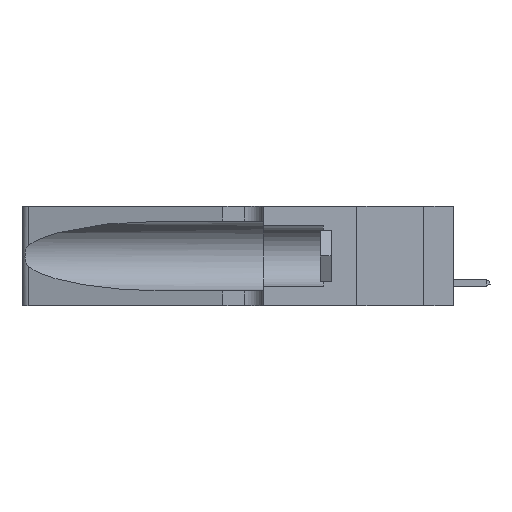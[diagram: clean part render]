
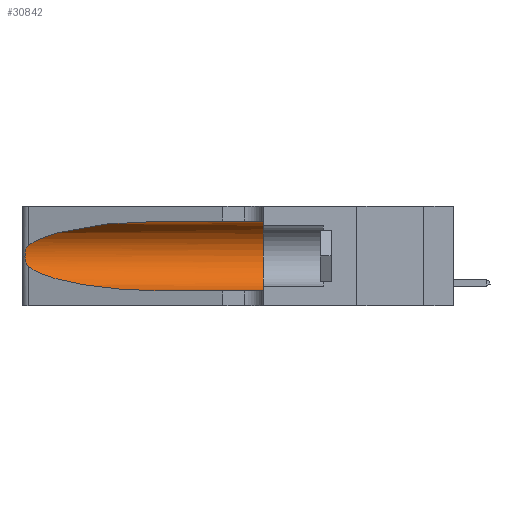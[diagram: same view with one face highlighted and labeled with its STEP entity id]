
A CAD part, left-side view. The second image highlights one B-rep face of the part: STEP entity #30842.
In plain terms, the highlighted cylindrical face has radius 3.308 mm (diameter 6.617 mm), a partial arc.
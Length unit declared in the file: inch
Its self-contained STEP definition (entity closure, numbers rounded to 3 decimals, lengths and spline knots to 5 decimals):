
#188 =( BOUNDED_CURVE ( )  B_SPLINE_CURVE ( 3, ( #22121, #29114, #4600, #29251 ),
 .UNSPECIFIED., .F., .F. ) 
 B_SPLINE_CURVE_WITH_KNOTS ( ( 4, 4 ),
 ( 3.44316, 4.71239 ),
 .UNSPECIFIED. ) 
 CURVE ( )  GEOMETRIC_REPRESENTATION_ITEM ( )  RATIONAL_B_SPLINE_CURVE ( ( 1., 0.87, 0.87, 1. ) ) 
 REPRESENTATION_ITEM ( '' )  );
#1077 = CARTESIAN_POINT ( 'NONE',  ( 0.25487, 1.22718, 0.22369 ) ) ;
#1195 = CYLINDRICAL_SURFACE ( 'NONE', #4130, 0.13025 ) ;
#1850 = CARTESIAN_POINT ( 'NONE',  ( 0.1305, 0.35, 0.31525 ) ) ;
#2791 = ORIENTED_EDGE ( 'NONE', *, *, #32027, .T. ) ;
#3034 = CARTESIAN_POINT ( 'NONE',  ( 0.25487, 1.22718, 0.14631 ) ) ;
#3228 = B_SPLINE_CURVE_WITH_KNOTS ( 'NONE', 3,
 ( #8041, #13827, #14368, #7908, #35420, #29452, #14245, #26494, #29583, #11113, #35843, #17309, #5080, #26637 ),
 .UNSPECIFIED., .F., .F.,
 ( 4, 2, 2, 2, 2, 2, 4 ),
 ( 0., 0.00027, 0.00053, 0.00107, 0.0016, 0.00187, 0.00214 ),
 .UNSPECIFIED. ) ;
#3767 = VERTEX_POINT ( 'NONE', #1850 ) ;
#4130 = AXIS2_PLACEMENT_3D ( 'NONE', #20902, #27401, #15110 ) ;
#4600 = CARTESIAN_POINT ( 'NONE',  ( 0.18966, 0.96281, 0.05475 ) ) ;
#5080 = CARTESIAN_POINT ( 'NONE',  ( 0.25555, 1.22993, 0.14849 ) ) ;
#5114 = EDGE_CURVE ( 'NONE', #3767, #33739, #23675, .T. ) ;
#5164 = CARTESIAN_POINT ( 'NONE',  ( 0.1305, 0.72297, 0.31525 ) ) ;
#5183 = CARTESIAN_POINT ( 'NONE',  ( 0.1305, 1.61858, 0.31525 ) ) ;
#5314 = DIRECTION ( 'NONE',  ( 0., -1., 0. ) ) ;
#5830 = AXIS2_PLACEMENT_3D ( 'NONE', #5868, #37039, #36783 ) ;
#5868 = CARTESIAN_POINT ( 'NONE',  ( 0.1305, 0.35, 0.185 ) ) ;
#7737 = ORIENTED_EDGE ( 'NONE', *, *, #20285, .F. ) ;
#7805 = EDGE_LOOP ( 'NONE', ( #2791, #36984, #19029, #29726, #11696, #7737 ) ) ;
#7908 = CARTESIAN_POINT ( 'NONE',  ( 0.25787, 1.23484, 0.2124 ) ) ;
#8041 = CARTESIAN_POINT ( 'NONE',  ( 0.25487, 1.22718, 0.22369 ) ) ;
#11113 = CARTESIAN_POINT ( 'NONE',  ( 0.25856, 1.23593, 0.16098 ) ) ;
#11696 = ORIENTED_EDGE ( 'NONE', *, *, #5114, .F. ) ;
#13827 = CARTESIAN_POINT ( 'NONE',  ( 0.25555, 1.22994, 0.2215 ) ) ;
#14245 = CARTESIAN_POINT ( 'NONE',  ( 0.26075, 1.23896, 0.19203 ) ) ;
#14368 = CARTESIAN_POINT ( 'NONE',  ( 0.25639, 1.23184, 0.21858 ) ) ;
#14747 = VECTOR ( 'NONE', #22527, 39.37008 ) ;
#14968 = CARTESIAN_POINT ( 'NONE',  ( 0.18966, 0.96281, 0.31525 ) ) ;
#15110 = DIRECTION ( 'NONE',  ( 0., 0., -1. ) ) ;
#15194 = LINE ( 'NONE', #20760, #14747 ) ;
#15802 = VECTOR ( 'NONE', #5314, 39.37008 ) ;
#17309 = CARTESIAN_POINT ( 'NONE',  ( 0.25639, 1.23186, 0.15144 ) ) ;
#19029 = ORIENTED_EDGE ( 'NONE', *, *, #26553, .T. ) ;
#20285 = EDGE_CURVE ( 'NONE', #37282, #3767, #34642, .T. ) ;
#20647 = VERTEX_POINT ( 'NONE', #37634 ) ;
#20760 = CARTESIAN_POINT ( 'NONE',  ( 0.1305, 1.61858, 0.05475 ) ) ;
#20902 = CARTESIAN_POINT ( 'NONE',  ( 0.1305, 1.61858, 0.185 ) ) ;
#22121 = CARTESIAN_POINT ( 'NONE',  ( 0.25487, 1.22718, 0.14631 ) ) ;
#22527 = DIRECTION ( 'NONE',  ( 0., -1., 0. ) ) ;
#23675 = CIRCLE ( 'NONE', #5830, 0.13025 ) ;
#24002 = CARTESIAN_POINT ( 'NONE',  ( 0.1305, 0.72297, 0.31525 ) ) ;
#26494 = CARTESIAN_POINT ( 'NONE',  ( 0.26075, 1.23896, 0.178 ) ) ;
#26553 = EDGE_CURVE ( 'NONE', #36859, #20647, #188, .T. ) ;
#26637 = CARTESIAN_POINT ( 'NONE',  ( 0.25487, 1.22718, 0.14631 ) ) ;
#27401 = DIRECTION ( 'NONE',  ( 0., -1., 0. ) ) ;
#28556 = EDGE_CURVE ( 'NONE', #35751, #36859, #3228, .T. ) ;
#29114 = CARTESIAN_POINT ( 'NONE',  ( 0.2373, 1.15595, 0.08982 ) ) ;
#29251 = CARTESIAN_POINT ( 'NONE',  ( 0.1305, 0.72297, 0.05475 ) ) ;
#29452 = CARTESIAN_POINT ( 'NONE',  ( 0.26018, 1.23835, 0.19895 ) ) ;
#29583 = CARTESIAN_POINT ( 'NONE',  ( 0.26017, 1.23833, 0.17102 ) ) ;
#29726 = ORIENTED_EDGE ( 'NONE', *, *, #31558, .T. ) ;
#30842 = ADVANCED_FACE ( 'NONE', ( #38981 ), #1195, .F. ) ;
#31558 = EDGE_CURVE ( 'NONE', #20647, #33739, #15194, .T. ) ;
#32027 = EDGE_CURVE ( 'NONE', #37282, #35751, #36159, .T. ) ;
#33739 = VERTEX_POINT ( 'NONE', #38639 ) ;
#34642 = LINE ( 'NONE', #5183, #15802 ) ;
#35420 = CARTESIAN_POINT ( 'NONE',  ( 0.25854, 1.2359, 0.20912 ) ) ;
#35751 = VERTEX_POINT ( 'NONE', #1077 ) ;
#35843 = CARTESIAN_POINT ( 'NONE',  ( 0.25789, 1.23486, 0.15765 ) ) ;
#36159 =( BOUNDED_CURVE ( )  B_SPLINE_CURVE ( 3, ( #24002, #14968, #36591, #36471 ),
 .UNSPECIFIED., .F., .F. ) 
 B_SPLINE_CURVE_WITH_KNOTS ( ( 4, 4 ),
 ( 1.5708, 2.84003 ),
 .UNSPECIFIED. ) 
 CURVE ( )  GEOMETRIC_REPRESENTATION_ITEM ( )  RATIONAL_B_SPLINE_CURVE ( ( 1., 0.87, 0.87, 1. ) ) 
 REPRESENTATION_ITEM ( '' )  );
#36471 = CARTESIAN_POINT ( 'NONE',  ( 0.25487, 1.22718, 0.22369 ) ) ;
#36591 = CARTESIAN_POINT ( 'NONE',  ( 0.2373, 1.15595, 0.28018 ) ) ;
#36783 = DIRECTION ( 'NONE',  ( 0., 0., 1. ) ) ;
#36859 = VERTEX_POINT ( 'NONE', #3034 ) ;
#36984 = ORIENTED_EDGE ( 'NONE', *, *, #28556, .T. ) ;
#37039 = DIRECTION ( 'NONE',  ( 0., 1., 0. ) ) ;
#37282 = VERTEX_POINT ( 'NONE', #5164 ) ;
#37634 = CARTESIAN_POINT ( 'NONE',  ( 0.1305, 0.72297, 0.05475 ) ) ;
#38639 = CARTESIAN_POINT ( 'NONE',  ( 0.1305, 0.35, 0.05475 ) ) ;
#38981 = FACE_OUTER_BOUND ( 'NONE', #7805, .T. ) ;
